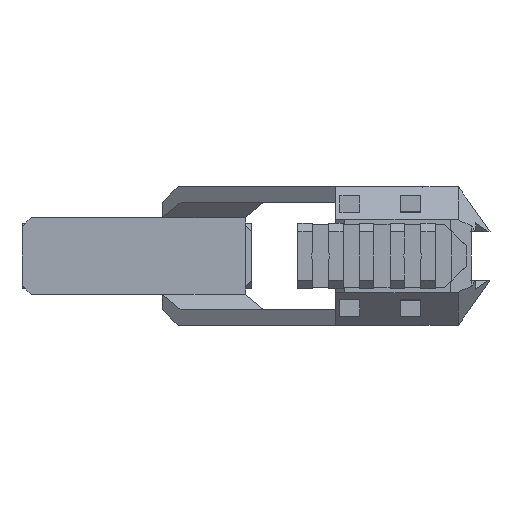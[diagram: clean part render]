
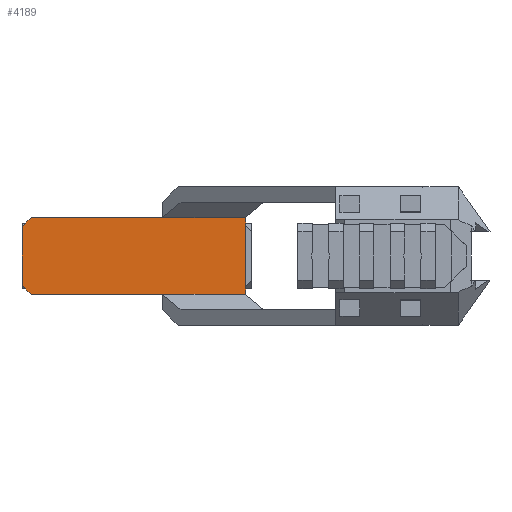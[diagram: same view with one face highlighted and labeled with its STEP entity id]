
A CAD part, front view. The second image highlights one B-rep face of the part: STEP entity #4189.
In plain terms, the highlighted planar face has unit normal (0, -1, 0).
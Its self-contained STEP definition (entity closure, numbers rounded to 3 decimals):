
#121=FACE_OUTER_BOUND('',#334,.T.);
#334=EDGE_LOOP('',(#3052,#3053,#3054,#3055,#3056,#3057,#3058,#3059,#3060,
#3061,#3062,#3063));
#702=LINE('',#6098,#1289);
#704=LINE('',#6103,#1291);
#708=LINE('',#6110,#1295);
#712=LINE('',#6118,#1299);
#745=LINE('',#6180,#1332);
#746=LINE('',#6182,#1333);
#747=LINE('',#6184,#1334);
#748=LINE('',#6186,#1335);
#749=LINE('',#6188,#1336);
#750=LINE('',#6189,#1337);
#751=LINE('',#6191,#1338);
#752=LINE('',#6192,#1339);
#1289=VECTOR('',#4902,10.);
#1291=VECTOR('',#4906,10.);
#1295=VECTOR('',#4912,10.);
#1299=VECTOR('',#4920,10.);
#1332=VECTOR('',#4971,10.);
#1333=VECTOR('',#4972,10.);
#1334=VECTOR('',#4973,10.);
#1335=VECTOR('',#4974,10.);
#1336=VECTOR('',#4975,10.);
#1337=VECTOR('',#4976,10.);
#1338=VECTOR('',#4977,10.);
#1339=VECTOR('',#4978,10.);
#1787=VERTEX_POINT('',#5962);
#1797=VERTEX_POINT('',#5984);
#1836=VERTEX_POINT('',#6092);
#1838=VERTEX_POINT('',#6096);
#1839=VERTEX_POINT('',#6100);
#1842=VERTEX_POINT('',#6108);
#1864=VERTEX_POINT('',#6179);
#1865=VERTEX_POINT('',#6181);
#1866=VERTEX_POINT('',#6183);
#1867=VERTEX_POINT('',#6185);
#1868=VERTEX_POINT('',#6187);
#1869=VERTEX_POINT('',#6190);
#2288=EDGE_CURVE('',#1836,#1838,#702,.T.);
#2290=EDGE_CURVE('',#1797,#1839,#704,.T.);
#2294=EDGE_CURVE('',#1797,#1842,#708,.T.);
#2298=EDGE_CURVE('',#1787,#1838,#712,.T.);
#2331=EDGE_CURVE('',#1864,#1842,#745,.T.);
#2332=EDGE_CURVE('',#1865,#1839,#746,.T.);
#2333=EDGE_CURVE('',#1865,#1866,#747,.T.);
#2334=EDGE_CURVE('',#1866,#1867,#748,.T.);
#2335=EDGE_CURVE('',#1867,#1868,#749,.T.);
#2336=EDGE_CURVE('',#1836,#1868,#750,.T.);
#2337=EDGE_CURVE('',#1787,#1869,#751,.T.);
#2338=EDGE_CURVE('',#1869,#1864,#752,.T.);
#3052=ORIENTED_EDGE('',*,*,#2331,.T.);
#3053=ORIENTED_EDGE('',*,*,#2294,.F.);
#3054=ORIENTED_EDGE('',*,*,#2290,.T.);
#3055=ORIENTED_EDGE('',*,*,#2332,.F.);
#3056=ORIENTED_EDGE('',*,*,#2333,.T.);
#3057=ORIENTED_EDGE('',*,*,#2334,.T.);
#3058=ORIENTED_EDGE('',*,*,#2335,.T.);
#3059=ORIENTED_EDGE('',*,*,#2336,.F.);
#3060=ORIENTED_EDGE('',*,*,#2288,.T.);
#3061=ORIENTED_EDGE('',*,*,#2298,.F.);
#3062=ORIENTED_EDGE('',*,*,#2337,.T.);
#3063=ORIENTED_EDGE('',*,*,#2338,.T.);
#3990=PLANE('',#4418);
#4189=ADVANCED_FACE('',(#121),#3990,.T.);
#4418=AXIS2_PLACEMENT_3D('',#6178,#4969,#4970);
#4902=DIRECTION('',(1.,0.,0.));
#4906=DIRECTION('',(-1.,0.,0.));
#4912=DIRECTION('',(1.,0.,0.));
#4920=DIRECTION('',(-1.,0.,0.));
#4969=DIRECTION('center_axis',(0.,-1.,0.));
#4970=DIRECTION('ref_axis',(1.,0.,0.));
#4971=DIRECTION('',(0.,0.,1.));
#4972=DIRECTION('',(0.707,0.,0.707));
#4973=DIRECTION('',(-0.707,0.,-0.707));
#4974=DIRECTION('',(0.,0.,-1.));
#4975=DIRECTION('',(0.707,0.,-0.707));
#4976=DIRECTION('',(-0.707,0.,0.707));
#4977=DIRECTION('',(0.,0.,1.));
#4978=DIRECTION('',(0.,0.,1.));
#5962=CARTESIAN_POINT('',(32.727,78.434,4.989));
#5984=CARTESIAN_POINT('',(5.779,78.434,30.011));
#6092=CARTESIAN_POINT('',(-37.,78.434,4.989));
#6096=CARTESIAN_POINT('',(5.779,78.434,4.989));
#6098=CARTESIAN_POINT('',(-3.638,78.434,4.989));
#6100=CARTESIAN_POINT('',(-37.,78.434,30.011));
#6103=CARTESIAN_POINT('',(-3.638,78.434,30.011));
#6108=CARTESIAN_POINT('',(32.727,78.434,30.011));
#6110=CARTESIAN_POINT('',(32.724,78.434,30.011));
#6118=CARTESIAN_POINT('',(19.25,78.434,4.989));
#6178=CARTESIAN_POINT('Origin',(-25.,78.434,-0.011));
#6179=CARTESIAN_POINT('',(32.727,78.434,27.5));
#6180=CARTESIAN_POINT('',(32.727,78.434,-0.011));
#6181=CARTESIAN_POINT('',(-39.511,78.434,27.5));
#6182=CARTESIAN_POINT('',(-42.256,78.434,24.756));
#6183=CARTESIAN_POINT('',(-40.,78.434,27.011));
#6184=CARTESIAN_POINT('',(-44.128,78.434,22.884));
#6185=CARTESIAN_POINT('',(-40.,78.434,7.989));
#6186=CARTESIAN_POINT('',(-40.,78.434,3.744));
#6187=CARTESIAN_POINT('',(-39.511,78.434,7.5));
#6188=CARTESIAN_POINT('',(-39.128,78.434,7.116));
#6189=CARTESIAN_POINT('',(-33.5,78.434,1.489));
#6190=CARTESIAN_POINT('',(32.727,78.434,7.5));
#6191=CARTESIAN_POINT('',(32.727,78.434,-0.011));
#6192=CARTESIAN_POINT('',(32.727,78.434,3.744));
